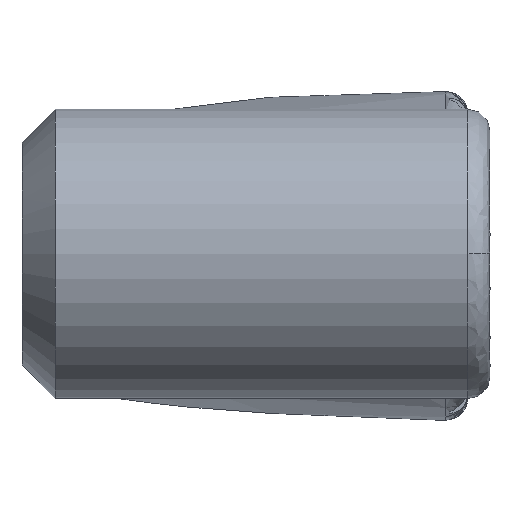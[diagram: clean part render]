
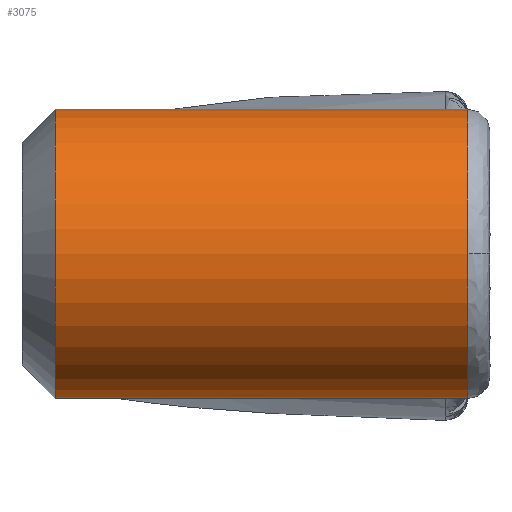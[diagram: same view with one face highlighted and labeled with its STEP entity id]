
A CAD part, top view. The second image highlights one B-rep face of the part: STEP entity #3075.
In plain terms, the highlighted cylindrical face has radius 6.5 mm (diameter 13 mm), a partial arc.
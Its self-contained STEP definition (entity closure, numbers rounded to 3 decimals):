
#164 = ORIENTED_EDGE ( 'NONE', *, *, #5750, .T. ) ;
#229 = DIRECTION ( 'NONE',  ( 0., -1., 0. ) ) ;
#267 = CARTESIAN_POINT ( 'NONE',  ( 80.679, 54.329, -20.721 ) ) ;
#307 = EDGE_CURVE ( 'NONE', #4312, #5330, #6192, .T. ) ;
#327 = AXIS2_PLACEMENT_3D ( 'NONE', #1859, #5634, #3056 ) ;
#572 = EDGE_CURVE ( 'NONE', #3970, #4312, #6515, .T. ) ;
#620 = DIRECTION ( 'NONE',  ( -1., 0., 0. ) ) ;
#641 = AXIS2_PLACEMENT_3D ( 'NONE', #1466, #6769, #3621 ) ;
#1165 = ORIENTED_EDGE ( 'NONE', *, *, #6046, .T. ) ;
#1397 = CYLINDRICAL_SURFACE ( 'NONE', #327, 6.5 ) ;
#1466 = CARTESIAN_POINT ( 'NONE',  ( 80.679, 47.829, -20.721 ) ) ;
#1539 = DIRECTION ( 'NONE',  ( 0., -1., 0. ) ) ;
#1859 = CARTESIAN_POINT ( 'NONE',  ( 75.679, 47.829, -20.721 ) ) ;
#1932 = VECTOR ( 'NONE', #620, 1000. ) ;
#1937 = ORIENTED_EDGE ( 'NONE', *, *, #307, .T. ) ;
#2345 = CARTESIAN_POINT ( 'NONE',  ( 62.179, 47.829, -20.721 ) ) ;
#2556 = CIRCLE ( 'NONE', #4935, 6.5 ) ;
#2800 = CARTESIAN_POINT ( 'NONE',  ( 75.679, 54.329, -20.721 ) ) ;
#2843 = CARTESIAN_POINT ( 'NONE',  ( 75.679, 41.329, -20.721 ) ) ;
#2916 = FACE_OUTER_BOUND ( 'NONE', #3448, .T. ) ;
#3056 = DIRECTION ( 'NONE',  ( 0., -1., 0. ) ) ;
#3060 = ORIENTED_EDGE ( 'NONE', *, *, #4195, .F. ) ;
#3075 = ADVANCED_FACE ( 'NONE', ( #2916 ), #1397, .T. ) ;
#3124 = ORIENTED_EDGE ( 'NONE', *, *, #572, .T. ) ;
#3417 = VERTEX_POINT ( 'NONE', #4921 ) ;
#3448 = EDGE_LOOP ( 'NONE', ( #1165, #164, #3124, #1937, #3060 ) ) ;
#3621 = DIRECTION ( 'NONE',  ( 0., -1., 0. ) ) ;
#3686 = CIRCLE ( 'NONE', #641, 6.5 ) ;
#3828 = VECTOR ( 'NONE', #4468, 1000. ) ;
#3970 = VERTEX_POINT ( 'NONE', #267 ) ;
#3976 = CARTESIAN_POINT ( 'NONE',  ( 80.679, 41.329, -20.721 ) ) ;
#4195 = EDGE_CURVE ( 'NONE', #5928, #5330, #5453, .T. ) ;
#4228 = DIRECTION ( 'NONE',  ( -1., 0., 0. ) ) ;
#4312 = VERTEX_POINT ( 'NONE', #6728 ) ;
#4468 = DIRECTION ( 'NONE',  ( -1., 0., 0. ) ) ;
#4921 = CARTESIAN_POINT ( 'NONE',  ( 80.679, 47.829, -14.221 ) ) ;
#4935 = AXIS2_PLACEMENT_3D ( 'NONE', #6918, #4228, #1539 ) ;
#5067 = DIRECTION ( 'NONE',  ( 1., 0., 0. ) ) ;
#5330 = VERTEX_POINT ( 'NONE', #6358 ) ;
#5453 = LINE ( 'NONE', #2843, #1932 ) ;
#5634 = DIRECTION ( 'NONE',  ( -1., 0., 0. ) ) ;
#5750 = EDGE_CURVE ( 'NONE', #3417, #3970, #2556, .T. ) ;
#5928 = VERTEX_POINT ( 'NONE', #3976 ) ;
#6046 = EDGE_CURVE ( 'NONE', #5928, #3417, #3686, .T. ) ;
#6192 = CIRCLE ( 'NONE', #6537, 6.5 ) ;
#6358 = CARTESIAN_POINT ( 'NONE',  ( 62.179, 41.329, -20.721 ) ) ;
#6515 = LINE ( 'NONE', #2800, #3828 ) ;
#6537 = AXIS2_PLACEMENT_3D ( 'NONE', #2345, #5067, #229 ) ;
#6728 = CARTESIAN_POINT ( 'NONE',  ( 62.179, 54.329, -20.721 ) ) ;
#6769 = DIRECTION ( 'NONE',  ( -1., 0., 0. ) ) ;
#6918 = CARTESIAN_POINT ( 'NONE',  ( 80.679, 47.829, -20.721 ) ) ;
